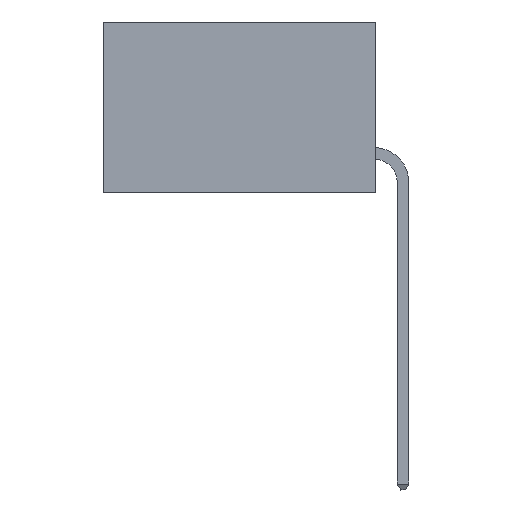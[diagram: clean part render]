
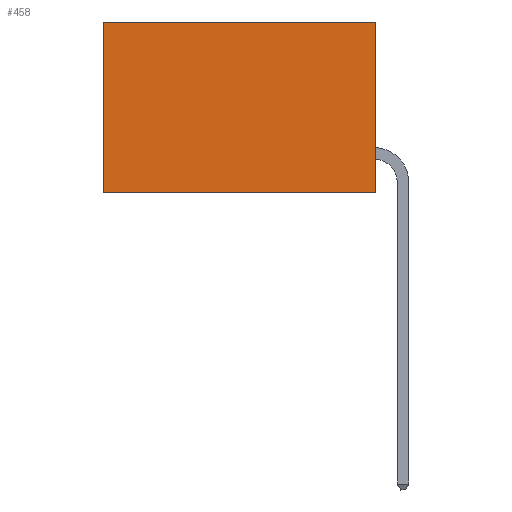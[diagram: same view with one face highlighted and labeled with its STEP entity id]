
A CAD part, left-side view. The second image highlights one B-rep face of the part: STEP entity #458.
In plain terms, the highlighted planar face has unit normal (-1, 0, 0).
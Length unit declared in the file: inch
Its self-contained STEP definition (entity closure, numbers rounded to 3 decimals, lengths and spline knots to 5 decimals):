
#24 = CARTESIAN_POINT ( 'NONE',  ( 0.277, 0.59, -0.37 ) ) ;
#52 = ORIENTED_EDGE ( 'NONE', *, *, #27556, .F. ) ;
#153 = VECTOR ( 'NONE', #2684, 39.37008 ) ;
#458 = ADVANCED_FACE ( 'NONE', ( #25933 ), #12041, .F. ) ;
#664 = ORIENTED_EDGE ( 'NONE', *, *, #2206, .F. ) ;
#905 = LINE ( 'NONE', #19446, #153 ) ;
#1365 = VERTEX_POINT ( 'NONE', #11661 ) ;
#1900 = ORIENTED_EDGE ( 'NONE', *, *, #29946, .T. ) ;
#2206 = EDGE_CURVE ( 'NONE', #9610, #4076, #7318, .T. ) ;
#2684 = DIRECTION ( 'NONE',  ( 0., 1., 0. ) ) ;
#4076 = VERTEX_POINT ( 'NONE', #22696 ) ;
#5287 = EDGE_CURVE ( 'NONE', #26869, #1365, #18670, .T. ) ;
#5405 = DIRECTION ( 'NONE',  ( 0., 0., -1. ) ) ;
#5959 = VECTOR ( 'NONE', #5405, 39.37008 ) ;
#7318 = LINE ( 'NONE', #13235, #18494 ) ;
#7584 = CARTESIAN_POINT ( 'NONE',  ( 0.277, 0.59, 0. ) ) ;
#7816 = CARTESIAN_POINT ( 'NONE',  ( 0.277, 0., -0.37 ) ) ;
#8266 = ORIENTED_EDGE ( 'NONE', *, *, #5287, .T. ) ;
#9610 = VERTEX_POINT ( 'NONE', #14881 ) ;
#10137 = DIRECTION ( 'NONE',  ( 0., 0., -1. ) ) ;
#10243 = DIRECTION ( 'NONE',  ( 0., 1., 0. ) ) ;
#11661 = CARTESIAN_POINT ( 'NONE',  ( 0.277, 0.59, -0.37 ) ) ;
#12041 = PLANE ( 'NONE',  #27220 ) ;
#13235 = CARTESIAN_POINT ( 'NONE',  ( 0.277, 0., -0.37 ) ) ;
#14881 = CARTESIAN_POINT ( 'NONE',  ( 0.277, 0., 0. ) ) ;
#15816 = DIRECTION ( 'NONE',  ( 0., 0., -1. ) ) ;
#18494 = VECTOR ( 'NONE', #15816, 39.37008 ) ;
#18670 = LINE ( 'NONE', #24, #5959 ) ;
#19019 = VECTOR ( 'NONE', #10243, 39.37008 ) ;
#19446 = CARTESIAN_POINT ( 'NONE',  ( 0.277, 0., 0. ) ) ;
#19774 = LINE ( 'NONE', #7816, #19019 ) ;
#22696 = CARTESIAN_POINT ( 'NONE',  ( 0.277, 0., -0.37 ) ) ;
#25143 = DIRECTION ( 'NONE',  ( 1., 0., 0. ) ) ;
#25179 = CARTESIAN_POINT ( 'NONE',  ( 0.277, 0., -0.37 ) ) ;
#25933 = FACE_OUTER_BOUND ( 'NONE', #28192, .T. ) ;
#26869 = VERTEX_POINT ( 'NONE', #7584 ) ;
#27220 = AXIS2_PLACEMENT_3D ( 'NONE', #25179, #25143, #10137 ) ;
#27556 = EDGE_CURVE ( 'NONE', #4076, #1365, #19774, .T. ) ;
#28192 = EDGE_LOOP ( 'NONE', ( #8266, #52, #664, #1900 ) ) ;
#29946 = EDGE_CURVE ( 'NONE', #9610, #26869, #905, .T. ) ;
